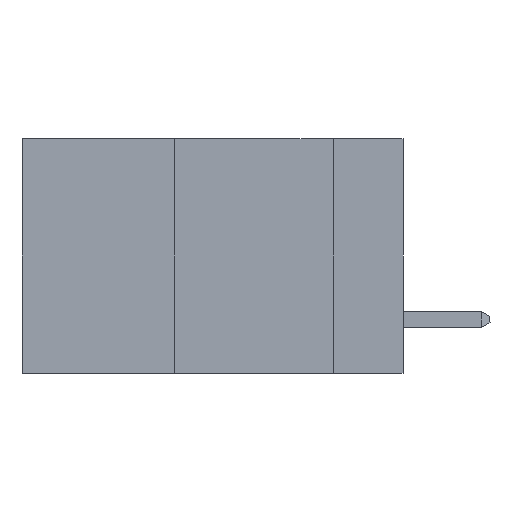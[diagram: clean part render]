
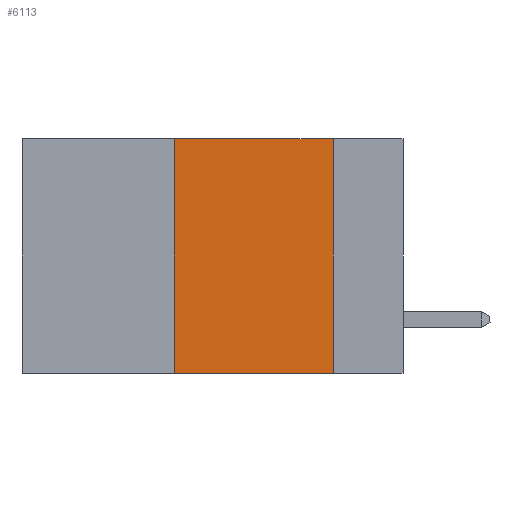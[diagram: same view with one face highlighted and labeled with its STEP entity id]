
A CAD part, left-side view. The second image highlights one B-rep face of the part: STEP entity #6113.
In plain terms, the highlighted planar face has unit normal (-1, 0, 0).
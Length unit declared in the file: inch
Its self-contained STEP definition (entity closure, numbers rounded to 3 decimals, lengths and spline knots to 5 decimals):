
#1008 = CARTESIAN_POINT ( 'NONE',  ( 0., 0.11, 0. ) ) ;
#1532 = VERTEX_POINT ( 'NONE', #14078 ) ;
#2244 = EDGE_CURVE ( 'NONE', #1532, #25253, #22343, .T. ) ;
#2567 = CARTESIAN_POINT ( 'NONE',  ( 0., 0.6, -0.37 ) ) ;
#3311 = DIRECTION ( 'NONE',  ( 0., 0., -1. ) ) ;
#3467 = VECTOR ( 'NONE', #3311, 39.37008 ) ;
#4657 = CARTESIAN_POINT ( 'NONE',  ( 0., 0.36, 0. ) ) ;
#4876 = CARTESIAN_POINT ( 'NONE',  ( 0., 0.11, -0.37 ) ) ;
#5265 = CARTESIAN_POINT ( 'NONE',  ( 0., 0.11, 0. ) ) ;
#6113 = ADVANCED_FACE ( 'NONE', ( #10148 ), #22473, .F. ) ;
#6976 = DIRECTION ( 'NONE',  ( 0., 0., 1. ) ) ;
#7323 = CARTESIAN_POINT ( 'NONE',  ( 0., 0.36, -0.37 ) ) ;
#9029 = CARTESIAN_POINT ( 'NONE',  ( 0., 0.6, 0. ) ) ;
#9416 = ORIENTED_EDGE ( 'NONE', *, *, #18491, .F. ) ;
#9521 = LINE ( 'NONE', #1008, #3467 ) ;
#10148 = FACE_OUTER_BOUND ( 'NONE', #13390, .T. ) ;
#10567 = VECTOR ( 'NONE', #20631, 39.37008 ) ;
#10978 = VECTOR ( 'NONE', #6976, 39.37008 ) ;
#11257 = LINE ( 'NONE', #2567, #10567 ) ;
#11273 = DIRECTION ( 'NONE',  ( 1., 0., 0. ) ) ;
#12438 = EDGE_CURVE ( 'NONE', #21234, #16031, #11257, .T. ) ;
#13390 = EDGE_LOOP ( 'NONE', ( #25218, #26640, #9416, #22076 ) ) ;
#14078 = CARTESIAN_POINT ( 'NONE',  ( 0., 0.36, 0. ) ) ;
#16031 = VERTEX_POINT ( 'NONE', #4876 ) ;
#18491 = EDGE_CURVE ( 'NONE', #21234, #1532, #28190, .T. ) ;
#20005 = EDGE_CURVE ( 'NONE', #25253, #16031, #9521, .T. ) ;
#20631 = DIRECTION ( 'NONE',  ( 0., -1., 0. ) ) ;
#21234 = VERTEX_POINT ( 'NONE', #7323 ) ;
#21315 = CARTESIAN_POINT ( 'NONE',  ( 0., 0.6, 0. ) ) ;
#21411 = DIRECTION ( 'NONE',  ( 0., -1., 0. ) ) ;
#22076 = ORIENTED_EDGE ( 'NONE', *, *, #12438, .T. ) ;
#22343 = LINE ( 'NONE', #21315, #27614 ) ;
#22473 = PLANE ( 'NONE',  #27054 ) ;
#25218 = ORIENTED_EDGE ( 'NONE', *, *, #20005, .F. ) ;
#25253 = VERTEX_POINT ( 'NONE', #5265 ) ;
#26640 = ORIENTED_EDGE ( 'NONE', *, *, #2244, .F. ) ;
#26996 = DIRECTION ( 'NONE',  ( 0., 0., -1. ) ) ;
#27054 = AXIS2_PLACEMENT_3D ( 'NONE', #9029, #11273, #26996 ) ;
#27614 = VECTOR ( 'NONE', #21411, 39.37008 ) ;
#28190 = LINE ( 'NONE', #4657, #10978 ) ;
